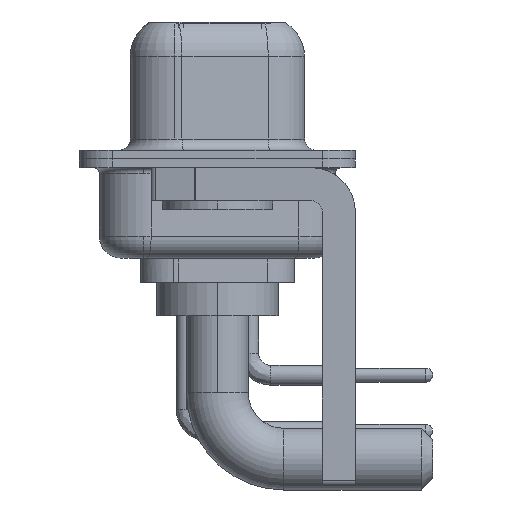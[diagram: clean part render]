
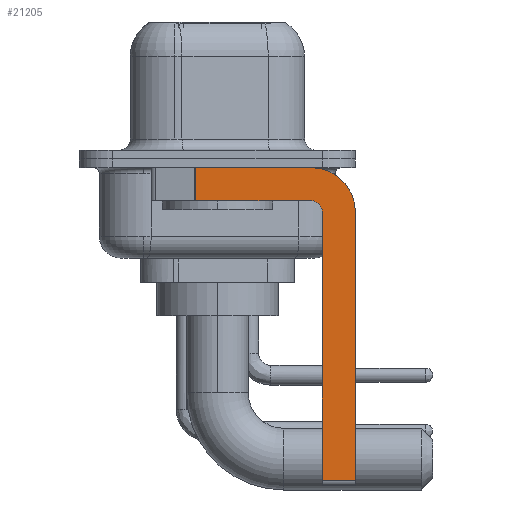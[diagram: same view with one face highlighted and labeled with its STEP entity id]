
A CAD part, left-side view. The second image highlights one B-rep face of the part: STEP entity #21205.
In plain terms, the highlighted planar face has unit normal (-1, 0, 0).
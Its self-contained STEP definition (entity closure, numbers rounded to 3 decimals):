
#400 = CARTESIAN_POINT ( 'NONE',  ( -2.9, 3., -0.4 ) ) ;
#457 = VERTEX_POINT ( 'NONE', #10014 ) ;
#746 = LINE ( 'NONE', #400, #16845 ) ;
#924 = DIRECTION ( 'NONE',  ( 1., 0., 0. ) ) ;
#1249 = CARTESIAN_POINT ( 'NONE',  ( -2.9, -4.25, -14.55 ) ) ;
#1508 = AXIS2_PLACEMENT_3D ( 'NONE', #21775, #924, #2757 ) ;
#1747 = VERTEX_POINT ( 'NONE', #5677 ) ;
#1997 = ORIENTED_EDGE ( 'NONE', *, *, #5104, .F. ) ;
#2448 = LINE ( 'NONE', #20203, #17618 ) ;
#2757 = DIRECTION ( 'NONE',  ( 0., 0., -1. ) ) ;
#4212 = CARTESIAN_POINT ( 'NONE',  ( -2.9, -4.25, -2.4 ) ) ;
#4372 = CIRCLE ( 'NONE', #10999, 0.5 ) ;
#4392 = DIRECTION ( 'NONE',  ( 1., 0., 0. ) ) ;
#4889 = CARTESIAN_POINT ( 'NONE',  ( -2.9, -6.25, -2.4 ) ) ;
#5095 = CARTESIAN_POINT ( 'NONE',  ( -2.9, -4.75, -2.4 ) ) ;
#5104 = EDGE_CURVE ( 'NONE', #22187, #19264, #5338, .T. ) ;
#5338 = LINE ( 'NONE', #4889, #15576 ) ;
#5677 = CARTESIAN_POINT ( 'NONE',  ( -2.9, 0.978, -1.9 ) ) ;
#5955 = DIRECTION ( 'NONE',  ( 0., 0., 1. ) ) ;
#6101 = CARTESIAN_POINT ( 'NONE',  ( -2.9, -4.25, -1.9 ) ) ;
#6239 = DIRECTION ( 'NONE',  ( 0., 0., -1. ) ) ;
#6390 = CIRCLE ( 'NONE', #19283, 2. ) ;
#6556 = LINE ( 'NONE', #15681, #8689 ) ;
#6956 = ORIENTED_EDGE ( 'NONE', *, *, #13621, .F. ) ;
#7477 = VECTOR ( 'NONE', #16501, 1000. ) ;
#7540 = EDGE_CURVE ( 'NONE', #15344, #1747, #9445, .T. ) ;
#8289 = DIRECTION ( 'NONE',  ( 0., -1., 0. ) ) ;
#8444 = EDGE_CURVE ( 'NONE', #21312, #22187, #6390, .T. ) ;
#8689 = VECTOR ( 'NONE', #13611, 1000. ) ;
#9445 = LINE ( 'NONE', #6101, #7477 ) ;
#9474 = CARTESIAN_POINT ( 'NONE',  ( -2.9, -6.25, -14.55 ) ) ;
#10013 = LINE ( 'NONE', #1249, #17551 ) ;
#10014 = CARTESIAN_POINT ( 'NONE',  ( -2.9, 0.978, -0.4 ) ) ;
#10268 = CARTESIAN_POINT ( 'NONE',  ( -2.9, -4.25, -0.4 ) ) ;
#10407 = EDGE_CURVE ( 'NONE', #12712, #19264, #10013, .T. ) ;
#10999 = AXIS2_PLACEMENT_3D ( 'NONE', #4212, #14852, #5955 ) ;
#11103 = CARTESIAN_POINT ( 'NONE',  ( -2.9, -4.25, -1.9 ) ) ;
#11560 = FACE_OUTER_BOUND ( 'NONE', #19624, .T. ) ;
#11636 = CARTESIAN_POINT ( 'NONE',  ( -2.9, -4.75, -14.55 ) ) ;
#11776 = EDGE_CURVE ( 'NONE', #457, #1747, #6556, .T. ) ;
#12499 = EDGE_CURVE ( 'NONE', #457, #21312, #746, .T. ) ;
#12515 = ORIENTED_EDGE ( 'NONE', *, *, #11776, .T. ) ;
#12712 = VERTEX_POINT ( 'NONE', #11636 ) ;
#12861 = ORIENTED_EDGE ( 'NONE', *, *, #12499, .F. ) ;
#13086 = DIRECTION ( 'NONE',  ( 0., 0., 1. ) ) ;
#13097 = ORIENTED_EDGE ( 'NONE', *, *, #10407, .T. ) ;
#13611 = DIRECTION ( 'NONE',  ( 0., 0., -1. ) ) ;
#13621 = EDGE_CURVE ( 'NONE', #12712, #16786, #2448, .T. ) ;
#14852 = DIRECTION ( 'NONE',  ( -1., 0., 0. ) ) ;
#15344 = VERTEX_POINT ( 'NONE', #11103 ) ;
#15576 = VECTOR ( 'NONE', #19415, 1000. ) ;
#15681 = CARTESIAN_POINT ( 'NONE',  ( -2.9, 0.978, -1.9 ) ) ;
#16501 = DIRECTION ( 'NONE',  ( 0., 1., 0. ) ) ;
#16738 = PLANE ( 'NONE',  #1508 ) ;
#16786 = VERTEX_POINT ( 'NONE', #5095 ) ;
#16845 = VECTOR ( 'NONE', #18271, 1000. ) ;
#17465 = ORIENTED_EDGE ( 'NONE', *, *, #8444, .F. ) ;
#17551 = VECTOR ( 'NONE', #8289, 1000. ) ;
#17618 = VECTOR ( 'NONE', #13086, 1000. ) ;
#17873 = EDGE_CURVE ( 'NONE', #16786, #15344, #4372, .T. ) ;
#18271 = DIRECTION ( 'NONE',  ( 0., -1., 0. ) ) ;
#18932 = ORIENTED_EDGE ( 'NONE', *, *, #17873, .F. ) ;
#19264 = VERTEX_POINT ( 'NONE', #9474 ) ;
#19283 = AXIS2_PLACEMENT_3D ( 'NONE', #20187, #4392, #6239 ) ;
#19415 = DIRECTION ( 'NONE',  ( 0., 0., -1. ) ) ;
#19624 = EDGE_LOOP ( 'NONE', ( #12861, #12515, #20150, #18932, #6956, #13097, #1997, #17465 ) ) ;
#20150 = ORIENTED_EDGE ( 'NONE', *, *, #7540, .F. ) ;
#20187 = CARTESIAN_POINT ( 'NONE',  ( -2.9, -4.25, -2.4 ) ) ;
#20203 = CARTESIAN_POINT ( 'NONE',  ( -2.9, -4.75, -14.8 ) ) ;
#21205 = ADVANCED_FACE ( 'NONE', ( #11560 ), #16738, .F. ) ;
#21312 = VERTEX_POINT ( 'NONE', #10268 ) ;
#21775 = CARTESIAN_POINT ( 'NONE',  ( -2.9, -4.25, -2.4 ) ) ;
#22187 = VERTEX_POINT ( 'NONE', #22658 ) ;
#22658 = CARTESIAN_POINT ( 'NONE',  ( -2.9, -6.25, -2.4 ) ) ;
